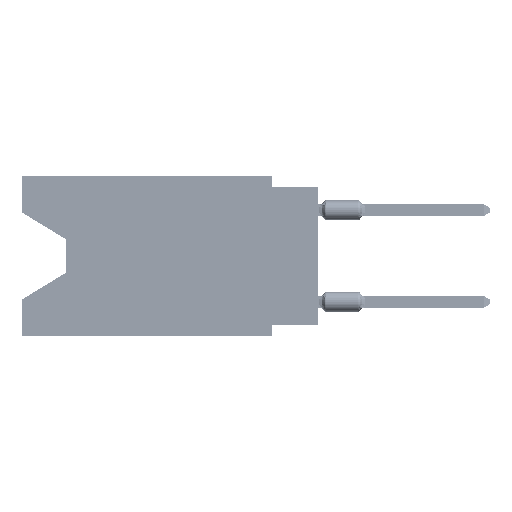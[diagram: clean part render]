
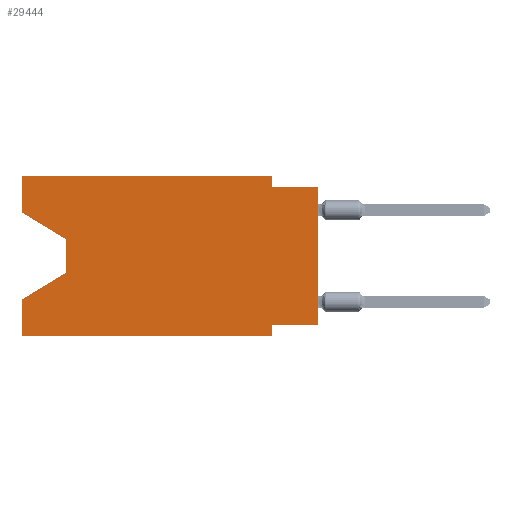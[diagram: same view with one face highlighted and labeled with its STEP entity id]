
A CAD part, left-side view. The second image highlights one B-rep face of the part: STEP entity #29444.
In plain terms, the highlighted planar face has unit normal (-1, 0, 0).
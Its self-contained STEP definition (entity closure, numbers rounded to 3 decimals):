
#1097 = EDGE_CURVE ( 'NONE', #19480, #116007, #13404, .T. ) ;
#2711 = DIRECTION ( 'NONE',  ( 0., 0., -1. ) ) ;
#2774 = CARTESIAN_POINT ( 'NONE',  ( 0., 2.54, -8.89 ) ) ;
#6426 = VERTEX_POINT ( 'NONE', #21493 ) ;
#6983 = LINE ( 'NONE', #42551, #116290 ) ;
#7321 = ORIENTED_EDGE ( 'NONE', *, *, #88643, .T. ) ;
#8176 = VECTOR ( 'NONE', #82826, 1000. ) ;
#8286 = CARTESIAN_POINT ( 'NONE',  ( 0., 13.97, -5.385 ) ) ;
#8572 = AXIS2_PLACEMENT_3D ( 'NONE', #20498, #19339, #2711 ) ;
#8591 = CARTESIAN_POINT ( 'NONE',  ( 0., 16.383, 0. ) ) ;
#9526 = ORIENTED_EDGE ( 'NONE', *, *, #103193, .F. ) ;
#9837 = LINE ( 'NONE', #45987, #46483 ) ;
#10104 = CARTESIAN_POINT ( 'NONE',  ( 0., 16.383, -2.038 ) ) ;
#10760 = DIRECTION ( 'NONE',  ( 0., 0., -1. ) ) ;
#12107 = VERTEX_POINT ( 'NONE', #8591 ) ;
#13404 = LINE ( 'NONE', #67344, #43819 ) ;
#15064 = ORIENTED_EDGE ( 'NONE', *, *, #106700, .T. ) ;
#19339 = DIRECTION ( 'NONE',  ( 1., 0., 0. ) ) ;
#19480 = VERTEX_POINT ( 'NONE', #102796 ) ;
#20498 = CARTESIAN_POINT ( 'NONE',  ( 0., 16.383, 0. ) ) ;
#20982 = CARTESIAN_POINT ( 'NONE',  ( 0., 2.54, -8.255 ) ) ;
#21176 = ORIENTED_EDGE ( 'NONE', *, *, #21423, .T. ) ;
#21423 = EDGE_CURVE ( 'NONE', #76443, #105137, #29678, .T. ) ;
#21493 = CARTESIAN_POINT ( 'NONE',  ( 0., 13.97, -3.505 ) ) ;
#21662 = PLANE ( 'NONE',  #8572 ) ;
#24087 = CARTESIAN_POINT ( 'NONE',  ( 0., 2.54, 0. ) ) ;
#24921 = DIRECTION ( 'NONE',  ( 0., 0.855, -0.519 ) ) ;
#26389 = VECTOR ( 'NONE', #10760, 1000. ) ;
#27839 = LINE ( 'NONE', #62825, #115865 ) ;
#29214 = ORIENTED_EDGE ( 'NONE', *, *, #40215, .F. ) ;
#29444 = ADVANCED_FACE ( 'NONE', ( #75587 ), #21662, .F. ) ;
#29678 = LINE ( 'NONE', #67590, #103135 ) ;
#35664 = CARTESIAN_POINT ( 'NONE',  ( 0., 0., -0.635 ) ) ;
#37092 = DIRECTION ( 'NONE',  ( 0., -1., 0. ) ) ;
#37112 = ORIENTED_EDGE ( 'NONE', *, *, #42961, .T. ) ;
#37376 = CARTESIAN_POINT ( 'NONE',  ( 0., 0., -8.255 ) ) ;
#38104 = LINE ( 'NONE', #74249, #42080 ) ;
#38357 = DIRECTION ( 'NONE',  ( 0., 0., -1. ) ) ;
#40215 = EDGE_CURVE ( 'NONE', #42693, #12107, #38104, .T. ) ;
#41103 = ORIENTED_EDGE ( 'NONE', *, *, #67927, .F. ) ;
#42080 = VECTOR ( 'NONE', #101496, 1000. ) ;
#42551 = CARTESIAN_POINT ( 'NONE',  ( 0., 0., -8.255 ) ) ;
#42693 = VERTEX_POINT ( 'NONE', #10104 ) ;
#42961 = EDGE_CURVE ( 'NONE', #19480, #96458, #72977, .T. ) ;
#43819 = VECTOR ( 'NONE', #67929, 1000. ) ;
#44338 = CARTESIAN_POINT ( 'NONE',  ( 0., 0., -0.635 ) ) ;
#45028 = ORIENTED_EDGE ( 'NONE', *, *, #1097, .F. ) ;
#45987 = CARTESIAN_POINT ( 'NONE',  ( 0., 16.383, 0. ) ) ;
#46483 = VECTOR ( 'NONE', #37092, 1000. ) ;
#48911 = CARTESIAN_POINT ( 'NONE',  ( 0., 13.97, -5.385 ) ) ;
#52086 = CARTESIAN_POINT ( 'NONE',  ( 0., 16.383, -8.89 ) ) ;
#59838 = DIRECTION ( 'NONE',  ( 0., 0., -1. ) ) ;
#61067 = LINE ( 'NONE', #8286, #73531 ) ;
#62825 = CARTESIAN_POINT ( 'NONE',  ( 0., 16.383, -2.038 ) ) ;
#66125 = EDGE_CURVE ( 'NONE', #86824, #96458, #100570, .T. ) ;
#67344 = CARTESIAN_POINT ( 'NONE',  ( 0., 16.383, 0. ) ) ;
#67467 = VERTEX_POINT ( 'NONE', #24087 ) ;
#67590 = CARTESIAN_POINT ( 'NONE',  ( 0., 0., 0. ) ) ;
#67927 = EDGE_CURVE ( 'NONE', #76443, #86824, #6983, .T. ) ;
#67929 = DIRECTION ( 'NONE',  ( 0., 0., 1. ) ) ;
#68250 = CARTESIAN_POINT ( 'NONE',  ( 0., 2.54, -0.635 ) ) ;
#72977 = LINE ( 'NONE', #52086, #87423 ) ;
#73531 = VECTOR ( 'NONE', #24921, 1000. ) ;
#73579 = LINE ( 'NONE', #108544, #26389 ) ;
#74046 = EDGE_CURVE ( 'NONE', #67467, #84515, #73579, .T. ) ;
#74249 = CARTESIAN_POINT ( 'NONE',  ( 0., 16.383, 0. ) ) ;
#75587 = FACE_OUTER_BOUND ( 'NONE', #117024, .T. ) ;
#76443 = VERTEX_POINT ( 'NONE', #37376 ) ;
#80314 = ORIENTED_EDGE ( 'NONE', *, *, #66125, .F. ) ;
#80493 = CARTESIAN_POINT ( 'NONE',  ( 0., 2.54, -8.89 ) ) ;
#82826 = DIRECTION ( 'NONE',  ( 0., -1., 0. ) ) ;
#83219 = EDGE_CURVE ( 'NONE', #84515, #105137, #99433, .T. ) ;
#84515 = VERTEX_POINT ( 'NONE', #68250 ) ;
#86824 = VERTEX_POINT ( 'NONE', #20982 ) ;
#87423 = VECTOR ( 'NONE', #115456, 1000. ) ;
#88643 = EDGE_CURVE ( 'NONE', #6426, #97007, #107188, .T. ) ;
#92518 = ORIENTED_EDGE ( 'NONE', *, *, #113326, .T. ) ;
#94902 = VECTOR ( 'NONE', #59838, 1000. ) ;
#96458 = VERTEX_POINT ( 'NONE', #80493 ) ;
#97007 = VERTEX_POINT ( 'NONE', #48911 ) ;
#97069 = DIRECTION ( 'NONE',  ( 0., 1., 0. ) ) ;
#97911 = ORIENTED_EDGE ( 'NONE', *, *, #83219, .F. ) ;
#98306 = CARTESIAN_POINT ( 'NONE',  ( 0., 13.97, -3.505 ) ) ;
#98361 = DIRECTION ( 'NONE',  ( 0., -0.855, -0.519 ) ) ;
#99433 = LINE ( 'NONE', #44338, #8176 ) ;
#100570 = LINE ( 'NONE', #2774, #107875 ) ;
#101496 = DIRECTION ( 'NONE',  ( 0., 0., 1. ) ) ;
#101736 = ORIENTED_EDGE ( 'NONE', *, *, #74046, .F. ) ;
#102796 = CARTESIAN_POINT ( 'NONE',  ( 0., 16.383, -8.89 ) ) ;
#103135 = VECTOR ( 'NONE', #112578, 1000. ) ;
#103193 = EDGE_CURVE ( 'NONE', #12107, #67467, #9837, .T. ) ;
#105137 = VERTEX_POINT ( 'NONE', #35664 ) ;
#106700 = EDGE_CURVE ( 'NONE', #97007, #116007, #61067, .T. ) ;
#107188 = LINE ( 'NONE', #98306, #94902 ) ;
#107875 = VECTOR ( 'NONE', #38357, 1000. ) ;
#108544 = CARTESIAN_POINT ( 'NONE',  ( 0., 2.54, 0. ) ) ;
#112578 = DIRECTION ( 'NONE',  ( 0., 0., 1. ) ) ;
#113253 = CARTESIAN_POINT ( 'NONE',  ( 0., 16.383, -6.852 ) ) ;
#113326 = EDGE_CURVE ( 'NONE', #42693, #6426, #27839, .T. ) ;
#115456 = DIRECTION ( 'NONE',  ( 0., -1., 0. ) ) ;
#115865 = VECTOR ( 'NONE', #98361, 1000. ) ;
#116007 = VERTEX_POINT ( 'NONE', #113253 ) ;
#116290 = VECTOR ( 'NONE', #97069, 1000. ) ;
#117024 = EDGE_LOOP ( 'NONE', ( #92518, #7321, #15064, #45028, #37112, #80314, #41103, #21176, #97911, #101736, #9526, #29214 ) ) ;
